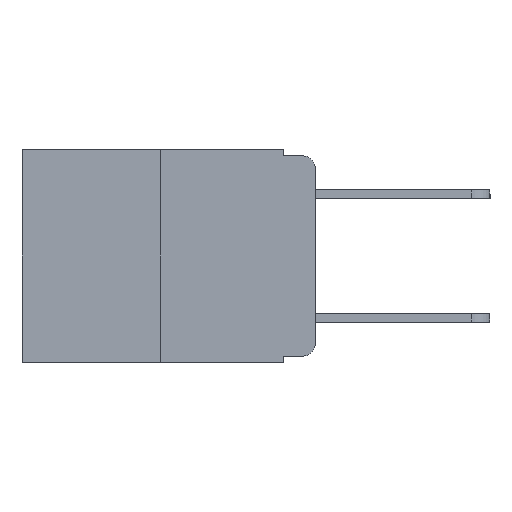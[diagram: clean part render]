
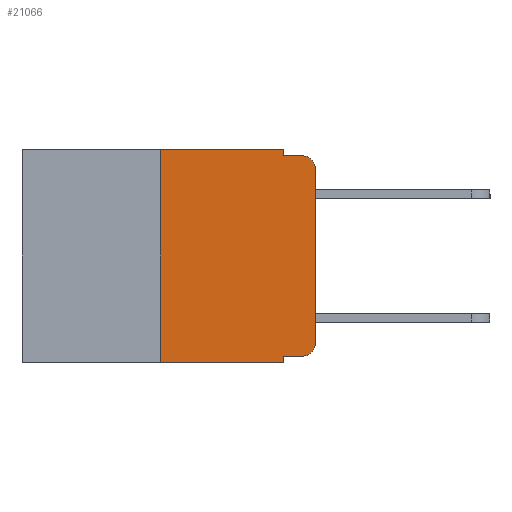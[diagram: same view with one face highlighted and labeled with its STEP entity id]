
A CAD part, left-side view. The second image highlights one B-rep face of the part: STEP entity #21066.
In plain terms, the highlighted planar face has unit normal (-1, 0, 0).
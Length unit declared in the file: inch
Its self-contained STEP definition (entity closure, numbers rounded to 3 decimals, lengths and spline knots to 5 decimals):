
#43 = LINE ( 'NONE', #12105, #23078 ) ;
#209 = EDGE_CURVE ( 'NONE', #20623, #3399, #11137, .T. ) ;
#210 = DIRECTION ( 'NONE',  ( 0., -1., 0. ) ) ;
#230 = CARTESIAN_POINT ( 'NONE',  ( 0., 0.02, -0.313 ) ) ;
#267 = VECTOR ( 'NONE', #14305, 39.37008 ) ;
#303 = CARTESIAN_POINT ( 'NONE',  ( 0., 0.051, -0.333 ) ) ;
#311 = CARTESIAN_POINT ( 'NONE',  ( 0., 0.473, 0. ) ) ;
#1018 = ORIENTED_EDGE ( 'NONE', *, *, #3841, .T. ) ;
#1149 = DIRECTION ( 'NONE',  ( 0., 0., -1. ) ) ;
#1522 = LINE ( 'NONE', #311, #11775 ) ;
#2091 = DIRECTION ( 'NONE',  ( 0., 0., -1. ) ) ;
#2731 = EDGE_CURVE ( 'NONE', #12852, #3399, #10187, .T. ) ;
#2892 = EDGE_CURVE ( 'NONE', #4851, #10863, #12149, .T. ) ;
#3141 = DIRECTION ( 'NONE',  ( 0., 0., -1. ) ) ;
#3395 = CARTESIAN_POINT ( 'NONE',  ( 0., 0., -0.313 ) ) ;
#3399 = VERTEX_POINT ( 'NONE', #8956 ) ;
#3657 = CARTESIAN_POINT ( 'NONE',  ( 0., 0.051, -0.01 ) ) ;
#3841 = EDGE_CURVE ( 'NONE', #21606, #16332, #8560, .T. ) ;
#4270 = CARTESIAN_POINT ( 'NONE',  ( 0., 0., -0.03 ) ) ;
#4613 = LINE ( 'NONE', #8881, #267 ) ;
#4827 = ORIENTED_EDGE ( 'NONE', *, *, #209, .T. ) ;
#4851 = VERTEX_POINT ( 'NONE', #23361 ) ;
#5261 = AXIS2_PLACEMENT_3D ( 'NONE', #15457, #20926, #10100 ) ;
#5932 = ORIENTED_EDGE ( 'NONE', *, *, #9097, .F. ) ;
#6017 = CARTESIAN_POINT ( 'NONE',  ( 0., 0.25, 0. ) ) ;
#6048 = VECTOR ( 'NONE', #16661, 39.37008 ) ;
#6337 = VECTOR ( 'NONE', #210, 39.37008 ) ;
#6596 = EDGE_CURVE ( 'NONE', #10863, #21606, #16589, .T. ) ;
#6782 = EDGE_LOOP ( 'NONE', ( #11546, #1018, #13294, #5932, #21242, #12737, #4827, #15577, #22085, #18978 ) ) ;
#7575 = EDGE_CURVE ( 'NONE', #19713, #12336, #1522, .T. ) ;
#7768 = LINE ( 'NONE', #13871, #10839 ) ;
#7874 = EDGE_CURVE ( 'NONE', #22423, #16332, #43, .T. ) ;
#8482 = DIRECTION ( 'NONE',  ( -1., 0., 0. ) ) ;
#8560 = CIRCLE ( 'NONE', #13207, 0.02 ) ;
#8881 = CARTESIAN_POINT ( 'NONE',  ( 0., 0.25, 0. ) ) ;
#8956 = CARTESIAN_POINT ( 'NONE',  ( 0., 0.051, -0.343 ) ) ;
#9097 = EDGE_CURVE ( 'NONE', #12336, #22423, #7768, .T. ) ;
#9335 = CARTESIAN_POINT ( 'NONE',  ( 0., 0.473, -0.343 ) ) ;
#10100 = DIRECTION ( 'NONE',  ( 0., 0., -1. ) ) ;
#10187 = LINE ( 'NONE', #14020, #16650 ) ;
#10839 = VECTOR ( 'NONE', #1149, 39.37008 ) ;
#10862 = LINE ( 'NONE', #303, #6048 ) ;
#10863 = VERTEX_POINT ( 'NONE', #3395 ) ;
#11137 = LINE ( 'NONE', #9335, #6337 ) ;
#11234 = DIRECTION ( 'NONE',  ( 0., -1., 0. ) ) ;
#11546 = ORIENTED_EDGE ( 'NONE', *, *, #6596, .T. ) ;
#11775 = VECTOR ( 'NONE', #11234, 39.37008 ) ;
#11822 = VECTOR ( 'NONE', #12074, 39.37008 ) ;
#12074 = DIRECTION ( 'NONE',  ( 0., 0., 1. ) ) ;
#12105 = CARTESIAN_POINT ( 'NONE',  ( 0., 0.051, -0.01 ) ) ;
#12149 = CIRCLE ( 'NONE', #13362, 0.02 ) ;
#12336 = VERTEX_POINT ( 'NONE', #18278 ) ;
#12351 = CARTESIAN_POINT ( 'NONE',  ( 0., 0.051, -0.333 ) ) ;
#12737 = ORIENTED_EDGE ( 'NONE', *, *, #19979, .F. ) ;
#12852 = VERTEX_POINT ( 'NONE', #12351 ) ;
#12983 = DIRECTION ( 'NONE',  ( -1., 0., 0. ) ) ;
#13064 = EDGE_CURVE ( 'NONE', #12852, #4851, #10862, .T. ) ;
#13207 = AXIS2_PLACEMENT_3D ( 'NONE', #19267, #8482, #21110 ) ;
#13294 = ORIENTED_EDGE ( 'NONE', *, *, #7874, .F. ) ;
#13362 = AXIS2_PLACEMENT_3D ( 'NONE', #230, #12983, #2091 ) ;
#13871 = CARTESIAN_POINT ( 'NONE',  ( 0., 0.051, 0. ) ) ;
#14020 = CARTESIAN_POINT ( 'NONE',  ( 0., 0.051, 0. ) ) ;
#14305 = DIRECTION ( 'NONE',  ( 0., 0., 1. ) ) ;
#14443 = FACE_OUTER_BOUND ( 'NONE', #6782, .T. ) ;
#15457 = CARTESIAN_POINT ( 'NONE',  ( 0., 0.473, 0. ) ) ;
#15577 = ORIENTED_EDGE ( 'NONE', *, *, #2731, .F. ) ;
#16332 = VERTEX_POINT ( 'NONE', #23303 ) ;
#16589 = LINE ( 'NONE', #17425, #11822 ) ;
#16650 = VECTOR ( 'NONE', #3141, 39.37008 ) ;
#16661 = DIRECTION ( 'NONE',  ( 0., -1., 0. ) ) ;
#17425 = CARTESIAN_POINT ( 'NONE',  ( 0., 0., 0. ) ) ;
#17834 = CARTESIAN_POINT ( 'NONE',  ( 0., 0.25, -0.343 ) ) ;
#18278 = CARTESIAN_POINT ( 'NONE',  ( 0., 0.051, 0. ) ) ;
#18978 = ORIENTED_EDGE ( 'NONE', *, *, #2892, .T. ) ;
#19086 = PLANE ( 'NONE',  #5261 ) ;
#19267 = CARTESIAN_POINT ( 'NONE',  ( 0., 0.02, -0.03 ) ) ;
#19288 = DIRECTION ( 'NONE',  ( 0., -1., 0. ) ) ;
#19713 = VERTEX_POINT ( 'NONE', #6017 ) ;
#19979 = EDGE_CURVE ( 'NONE', #20623, #19713, #4613, .T. ) ;
#20623 = VERTEX_POINT ( 'NONE', #17834 ) ;
#20926 = DIRECTION ( 'NONE',  ( 1., 0., 0. ) ) ;
#21066 = ADVANCED_FACE ( 'NONE', ( #14443 ), #19086, .F. ) ;
#21110 = DIRECTION ( 'NONE',  ( 0., 0., -1. ) ) ;
#21242 = ORIENTED_EDGE ( 'NONE', *, *, #7575, .F. ) ;
#21606 = VERTEX_POINT ( 'NONE', #4270 ) ;
#22085 = ORIENTED_EDGE ( 'NONE', *, *, #13064, .T. ) ;
#22423 = VERTEX_POINT ( 'NONE', #3657 ) ;
#23078 = VECTOR ( 'NONE', #19288, 39.37008 ) ;
#23303 = CARTESIAN_POINT ( 'NONE',  ( 0., 0.02, -0.01 ) ) ;
#23361 = CARTESIAN_POINT ( 'NONE',  ( 0., 0.02, -0.333 ) ) ;
